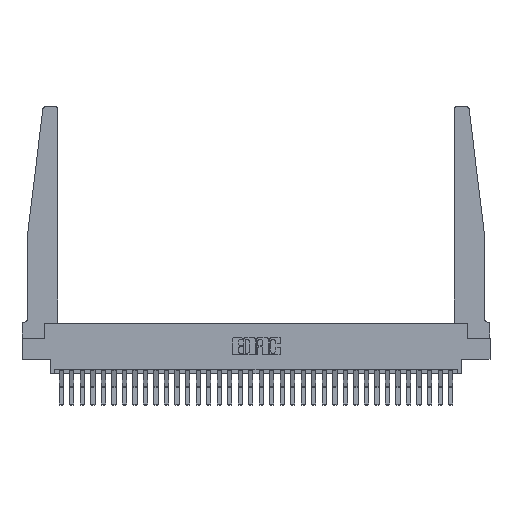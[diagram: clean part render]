
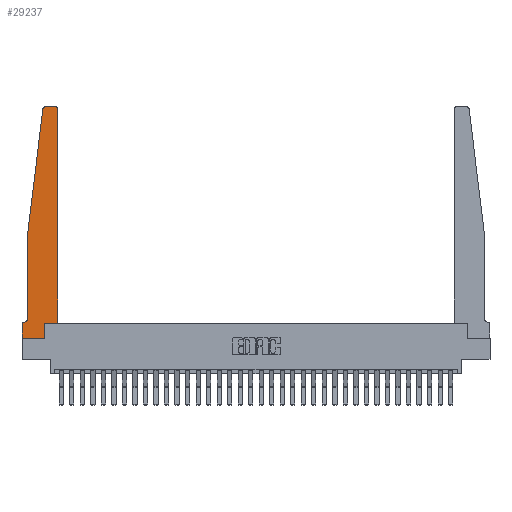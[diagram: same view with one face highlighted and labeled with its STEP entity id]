
A CAD part, top view. The second image highlights one B-rep face of the part: STEP entity #29237.
In plain terms, the highlighted planar face has unit normal (0, 0, 1).
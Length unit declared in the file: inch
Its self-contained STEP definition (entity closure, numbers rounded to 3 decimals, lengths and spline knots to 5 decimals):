
#77 = DIRECTION ( 'NONE',  ( 0., 0., 1. ) ) ;
#491 = EDGE_CURVE ( 'NONE', #19758, #7364, #22552, .T. ) ;
#1119 = LINE ( 'NONE', #19634, #26041 ) ;
#1313 = VECTOR ( 'NONE', #23055, 39.37008 ) ;
#1756 = CARTESIAN_POINT ( 'NONE',  ( 0.065, 0.1875, 0.37 ) ) ;
#1806 = CARTESIAN_POINT ( 'NONE',  ( 0.27653, 2.75, 0.37 ) ) ;
#1939 = CARTESIAN_POINT ( 'NONE',  ( 0.25, 2.75, 0.37 ) ) ;
#2195 = ORIENTED_EDGE ( 'NONE', *, *, #28695, .T. ) ;
#2217 = VERTEX_POINT ( 'NONE', #2607 ) ;
#2607 = CARTESIAN_POINT ( 'NONE',  ( 0.395, 2.75, 0.37 ) ) ;
#2826 = EDGE_LOOP ( 'NONE', ( #3641, #2878, #20542, #28170, #18690, #18720, #17572, #19563, #2195, #9144, #12787, #6613 ) ) ;
#2878 = ORIENTED_EDGE ( 'NONE', *, *, #29739, .T. ) ;
#3221 = DIRECTION ( 'NONE',  ( 0., -1., 0. ) ) ;
#3301 = CARTESIAN_POINT ( 'NONE',  ( 0.395, 2.72, 0.37 ) ) ;
#3641 = ORIENTED_EDGE ( 'NONE', *, *, #8966, .T. ) ;
#3832 = VECTOR ( 'NONE', #20419, 39.37008 ) ;
#4569 = VECTOR ( 'NONE', #30197, 39.37008 ) ;
#4922 = VERTEX_POINT ( 'NONE', #26888 ) ;
#5384 = CARTESIAN_POINT ( 'NONE',  ( 0.425, 0.18, 0.37 ) ) ;
#5659 = DIRECTION ( 'NONE',  ( 1., 0., 0. ) ) ;
#5852 = CARTESIAN_POINT ( 'NONE',  ( 0.425, 0.18, 0.37 ) ) ;
#6146 = AXIS2_PLACEMENT_3D ( 'NONE', #14202, #77, #16561 ) ;
#6420 = CARTESIAN_POINT ( 'NONE',  ( 0.2605, 0.18, 0.37 ) ) ;
#6591 = VERTEX_POINT ( 'NONE', #12537 ) ;
#6613 = ORIENTED_EDGE ( 'NONE', *, *, #28186, .T. ) ;
#6929 = VECTOR ( 'NONE', #14847, 39.37008 ) ;
#7249 = CARTESIAN_POINT ( 'NONE',  ( 0.2605, 0.18, 0.37 ) ) ;
#7364 = VERTEX_POINT ( 'NONE', #8299 ) ;
#7982 = EDGE_CURVE ( 'NONE', #20182, #16282, #19377, .T. ) ;
#8299 = CARTESIAN_POINT ( 'NONE',  ( 0., 0.1875, 0.37 ) ) ;
#8584 = EDGE_CURVE ( 'NONE', #25797, #4922, #10898, .T. ) ;
#8966 = EDGE_CURVE ( 'NONE', #2217, #27196, #25519, .T. ) ;
#9144 = ORIENTED_EDGE ( 'NONE', *, *, #27559, .T. ) ;
#9500 = CARTESIAN_POINT ( 'NONE',  ( 0.065, 1.25, 0.37 ) ) ;
#9627 = DIRECTION ( 'NONE',  ( 0., 1., 0. ) ) ;
#10042 = AXIS2_PLACEMENT_3D ( 'NONE', #3301, #19706, #5659 ) ;
#10056 = LINE ( 'NONE', #16264, #4569 ) ;
#10615 = CARTESIAN_POINT ( 'NONE',  ( 0.015, 0.2375, 0.37 ) ) ;
#10898 = LINE ( 'NONE', #14696, #16424 ) ;
#12159 = DIRECTION ( 'NONE',  ( 1., 0., 0. ) ) ;
#12537 = CARTESIAN_POINT ( 'NONE',  ( 0.24675, 2.72367, 0.37 ) ) ;
#12787 = ORIENTED_EDGE ( 'NONE', *, *, #13714, .T. ) ;
#12975 = DIRECTION ( 'NONE',  ( -1., 0., 0. ) ) ;
#13112 = EDGE_CURVE ( 'NONE', #6591, #20182, #26187, .T. ) ;
#13148 = VECTOR ( 'NONE', #24857, 39.37008 ) ;
#13714 = EDGE_CURVE ( 'NONE', #16824, #21302, #10056, .T. ) ;
#14202 = CARTESIAN_POINT ( 'NONE',  ( 0.27653, 2.72, 0.37 ) ) ;
#14696 = CARTESIAN_POINT ( 'NONE',  ( 0., 0., 0.37 ) ) ;
#14847 = DIRECTION ( 'NONE',  ( 1., 0., 0. ) ) ;
#15264 = VECTOR ( 'NONE', #23555, 39.37008 ) ;
#16026 = FACE_OUTER_BOUND ( 'NONE', #2826, .T. ) ;
#16264 = CARTESIAN_POINT ( 'NONE',  ( 0.425, 0.18, 0.37 ) ) ;
#16282 = VERTEX_POINT ( 'NONE', #24828 ) ;
#16424 = VECTOR ( 'NONE', #17058, 39.37008 ) ;
#16561 = DIRECTION ( 'NONE',  ( 1., 0., 0. ) ) ;
#16808 = CARTESIAN_POINT ( 'NONE',  ( 0., 0.1875, 0.37 ) ) ;
#16824 = VERTEX_POINT ( 'NONE', #5852 ) ;
#16956 = CARTESIAN_POINT ( 'NONE',  ( 0.425, 2.72, 0.37 ) ) ;
#17058 = DIRECTION ( 'NONE',  ( 1., 0., 0. ) ) ;
#17572 = ORIENTED_EDGE ( 'NONE', *, *, #20765, .T. ) ;
#18690 = ORIENTED_EDGE ( 'NONE', *, *, #23533, .T. ) ;
#18720 = ORIENTED_EDGE ( 'NONE', *, *, #491, .T. ) ;
#19377 = LINE ( 'NONE', #20172, #13148 ) ;
#19563 = ORIENTED_EDGE ( 'NONE', *, *, #8584, .T. ) ;
#19634 = CARTESIAN_POINT ( 'NONE',  ( 0., 0., 0.37 ) ) ;
#19706 = DIRECTION ( 'NONE',  ( 0., 0., 1. ) ) ;
#19758 = VERTEX_POINT ( 'NONE', #27783 ) ;
#20128 = VECTOR ( 'NONE', #9627, 39.37008 ) ;
#20172 = CARTESIAN_POINT ( 'NONE',  ( 0.065, 1.25, 0.37 ) ) ;
#20182 = VERTEX_POINT ( 'NONE', #24050 ) ;
#20248 = CARTESIAN_POINT ( 'NONE',  ( 0., 0., 0.37 ) ) ;
#20419 = DIRECTION ( 'NONE',  ( -1., 0., 0. ) ) ;
#20542 = ORIENTED_EDGE ( 'NONE', *, *, #13112, .T. ) ;
#20765 = EDGE_CURVE ( 'NONE', #7364, #25797, #1119, .T. ) ;
#20839 = LINE ( 'NONE', #7249, #20128 ) ;
#21302 = VERTEX_POINT ( 'NONE', #16956 ) ;
#21608 = CIRCLE ( 'NONE', #10042, 0.03 ) ;
#22313 = VERTEX_POINT ( 'NONE', #6420 ) ;
#22552 = LINE ( 'NONE', #1756, #3832 ) ;
#23055 = DIRECTION ( 'NONE',  ( -1., 0., 0. ) ) ;
#23369 = CIRCLE ( 'NONE', #6146, 0.03 ) ;
#23533 = EDGE_CURVE ( 'NONE', #16282, #19758, #25494, .T. ) ;
#23555 = DIRECTION ( 'NONE',  ( -0.122, -0.992, 0. ) ) ;
#23864 = PLANE ( 'NONE',  #24587 ) ;
#24050 = CARTESIAN_POINT ( 'NONE',  ( 0.065, 1.25, 0.37 ) ) ;
#24587 = AXIS2_PLACEMENT_3D ( 'NONE', #16808, #26163, #12159 ) ;
#24828 = CARTESIAN_POINT ( 'NONE',  ( 0.065, 0.2375, 0.37 ) ) ;
#24857 = DIRECTION ( 'NONE',  ( 0., -1., 0. ) ) ;
#25494 = CIRCLE ( 'NONE', #26032, 0.05 ) ;
#25519 = LINE ( 'NONE', #1939, #1313 ) ;
#25607 = LINE ( 'NONE', #5384, #6929 ) ;
#25797 = VERTEX_POINT ( 'NONE', #20248 ) ;
#26032 = AXIS2_PLACEMENT_3D ( 'NONE', #10615, #26968, #12975 ) ;
#26041 = VECTOR ( 'NONE', #3221, 39.37008 ) ;
#26163 = DIRECTION ( 'NONE',  ( 0., 0., 1. ) ) ;
#26187 = LINE ( 'NONE', #9500, #15264 ) ;
#26888 = CARTESIAN_POINT ( 'NONE',  ( 0.2605, 0., 0.37 ) ) ;
#26968 = DIRECTION ( 'NONE',  ( 0., 0., -1. ) ) ;
#27196 = VERTEX_POINT ( 'NONE', #1806 ) ;
#27559 = EDGE_CURVE ( 'NONE', #22313, #16824, #25607, .T. ) ;
#27783 = CARTESIAN_POINT ( 'NONE',  ( 0.015, 0.1875, 0.37 ) ) ;
#28170 = ORIENTED_EDGE ( 'NONE', *, *, #7982, .T. ) ;
#28186 = EDGE_CURVE ( 'NONE', #21302, #2217, #21608, .T. ) ;
#28695 = EDGE_CURVE ( 'NONE', #4922, #22313, #20839, .T. ) ;
#29237 = ADVANCED_FACE ( 'NONE', ( #16026 ), #23864, .T. ) ;
#29739 = EDGE_CURVE ( 'NONE', #27196, #6591, #23369, .T. ) ;
#30197 = DIRECTION ( 'NONE',  ( 0., 1., 0. ) ) ;
